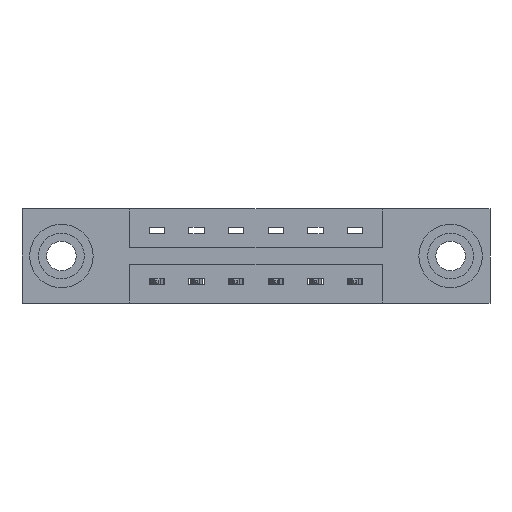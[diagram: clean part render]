
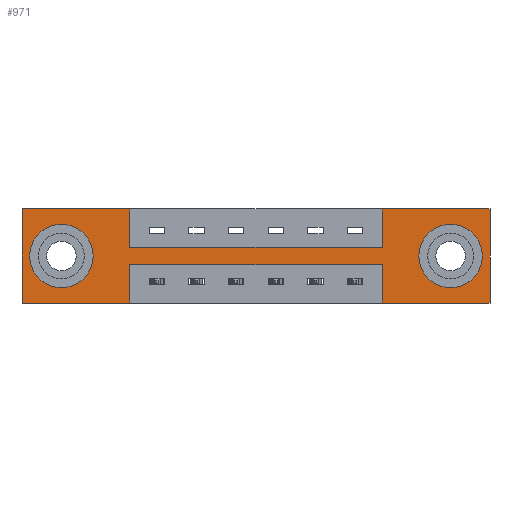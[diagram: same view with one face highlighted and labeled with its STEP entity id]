
A CAD part, front view. The second image highlights one B-rep face of the part: STEP entity #971.
In plain terms, the highlighted planar face has unit normal (0, -1, 0).
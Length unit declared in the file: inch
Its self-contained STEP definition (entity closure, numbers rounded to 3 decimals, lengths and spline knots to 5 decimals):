
#93 = VERTEX_POINT ( 'NONE', #6717 ) ;
#382 = ORIENTED_EDGE ( 'NONE', *, *, #2997, .F. ) ;
#542 = CARTESIAN_POINT ( 'NONE',  ( 1.417, 0., -0.15 ) ) ;
#563 = CARTESIAN_POINT ( 'NONE',  ( 0., 0., 0. ) ) ;
#632 = ORIENTED_EDGE ( 'NONE', *, *, #7686, .F. ) ;
#681 = EDGE_CURVE ( 'NONE', #6201, #2910, #5666, .T. ) ;
#719 = VERTEX_POINT ( 'NONE', #2175 ) ;
#766 = VERTEX_POINT ( 'NONE', #2208 ) ;
#838 = CIRCLE ( 'NONE', #7236, 0.078 ) ;
#924 = DIRECTION ( 'NONE',  ( 0., 0., -1. ) ) ;
#966 = CARTESIAN_POINT ( 'NONE',  ( 0., 0., -0.37 ) ) ;
#971 = ADVANCED_FACE ( 'NONE', ( #6395, #4572, #4335 ), #6551, .T. ) ;
#978 = LINE ( 'NONE', #7588, #6857 ) ;
#1150 = ORIENTED_EDGE ( 'NONE', *, *, #3278, .F. ) ;
#1361 = CARTESIAN_POINT ( 'NONE',  ( 0., 0., -0.37 ) ) ;
#1378 = VECTOR ( 'NONE', #2940, 39.37008 ) ;
#1530 = VECTOR ( 'NONE', #6991, 39.37008 ) ;
#1638 = VERTEX_POINT ( 'NONE', #3709 ) ;
#1661 = LINE ( 'NONE', #4416, #9433 ) ;
#1766 = VERTEX_POINT ( 'NONE', #563 ) ;
#1790 = ORIENTED_EDGE ( 'NONE', *, *, #7846, .T. ) ;
#2175 = CARTESIAN_POINT ( 'NONE',  ( 1.687, 0., -0.263 ) ) ;
#2208 = CARTESIAN_POINT ( 'NONE',  ( 0.425, 0., 0. ) ) ;
#2293 = VERTEX_POINT ( 'NONE', #4130 ) ;
#2416 = EDGE_CURVE ( 'NONE', #2293, #6888, #8305, .T. ) ;
#2449 = CARTESIAN_POINT ( 'NONE',  ( 1.687, 0., -0.185 ) ) ;
#2463 = CARTESIAN_POINT ( 'NONE',  ( 0.425, 0., 0. ) ) ;
#2646 = AXIS2_PLACEMENT_3D ( 'NONE', #8752, #4324, #9382 ) ;
#2883 = VERTEX_POINT ( 'NONE', #5233 ) ;
#2889 = CARTESIAN_POINT ( 'NONE',  ( 0.425, 0., -0.37 ) ) ;
#2910 = VERTEX_POINT ( 'NONE', #4475 ) ;
#2940 = DIRECTION ( 'NONE',  ( 0., 0., -1. ) ) ;
#2997 = EDGE_CURVE ( 'NONE', #1638, #3230, #7172, .T. ) ;
#3005 = LINE ( 'NONE', #4258, #5102 ) ;
#3043 = DIRECTION ( 'NONE',  ( 0., 1., 0. ) ) ;
#3058 = VECTOR ( 'NONE', #3884, 39.37008 ) ;
#3084 = LINE ( 'NONE', #4620, #8620 ) ;
#3142 = ORIENTED_EDGE ( 'NONE', *, *, #7053, .F. ) ;
#3230 = VERTEX_POINT ( 'NONE', #4614 ) ;
#3278 = EDGE_CURVE ( 'NONE', #2910, #93, #7640, .T. ) ;
#3315 = DIRECTION ( 'NONE',  ( 0., 0., -1. ) ) ;
#3488 = VERTEX_POINT ( 'NONE', #7374 ) ;
#3643 = CARTESIAN_POINT ( 'NONE',  ( 0.425, 0., -0.15 ) ) ;
#3709 = CARTESIAN_POINT ( 'NONE',  ( 1.842, 0., -0.37 ) ) ;
#3752 = LINE ( 'NONE', #9017, #9332 ) ;
#3884 = DIRECTION ( 'NONE',  ( -1., 0., 0. ) ) ;
#4019 = ORIENTED_EDGE ( 'NONE', *, *, #9321, .T. ) ;
#4111 = CIRCLE ( 'NONE', #8844, 0.078 ) ;
#4130 = CARTESIAN_POINT ( 'NONE',  ( 0.425, 0., -0.15 ) ) ;
#4258 = CARTESIAN_POINT ( 'NONE',  ( 1.842, 0., 0. ) ) ;
#4324 = DIRECTION ( 'NONE',  ( 0., 1., 0. ) ) ;
#4335 = FACE_OUTER_BOUND ( 'NONE', #8617, .T. ) ;
#4416 = CARTESIAN_POINT ( 'NONE',  ( 0., 0., 0. ) ) ;
#4475 = CARTESIAN_POINT ( 'NONE',  ( 0.425, 0., -0.37 ) ) ;
#4486 = ORIENTED_EDGE ( 'NONE', *, *, #8259, .F. ) ;
#4570 = CARTESIAN_POINT ( 'NONE',  ( 0.155, 0., -0.107 ) ) ;
#4572 = FACE_BOUND ( 'NONE', #6260, .T. ) ;
#4614 = CARTESIAN_POINT ( 'NONE',  ( 1.417, 0., -0.37 ) ) ;
#4620 = CARTESIAN_POINT ( 'NONE',  ( 0., 0., 0. ) ) ;
#4646 = CARTESIAN_POINT ( 'NONE',  ( 0.155, 0., -0.185 ) ) ;
#4681 = EDGE_CURVE ( 'NONE', #8097, #1638, #3005, .T. ) ;
#4729 = ORIENTED_EDGE ( 'NONE', *, *, #4681, .F. ) ;
#4920 = AXIS2_PLACEMENT_3D ( 'NONE', #4646, #9637, #5434 ) ;
#5102 = VECTOR ( 'NONE', #924, 39.37008 ) ;
#5192 = DIRECTION ( 'NONE',  ( 0., 0., 1. ) ) ;
#5233 = CARTESIAN_POINT ( 'NONE',  ( 1.417, 0., -0.22 ) ) ;
#5306 = EDGE_CURVE ( 'NONE', #93, #1766, #1661, .T. ) ;
#5434 = DIRECTION ( 'NONE',  ( 0., 0., 1. ) ) ;
#5518 = EDGE_CURVE ( 'NONE', #7432, #8097, #7824, .T. ) ;
#5534 = AXIS2_PLACEMENT_3D ( 'NONE', #966, #6732, #7203 ) ;
#5666 = LINE ( 'NONE', #2889, #1378 ) ;
#5799 = VECTOR ( 'NONE', #9416, 39.37008 ) ;
#5959 = VERTEX_POINT ( 'NONE', #6008 ) ;
#6008 = CARTESIAN_POINT ( 'NONE',  ( 0.155, 0., -0.263 ) ) ;
#6182 = DIRECTION ( 'NONE',  ( 1., 0., 0. ) ) ;
#6201 = VERTEX_POINT ( 'NONE', #7840 ) ;
#6251 = CARTESIAN_POINT ( 'NONE',  ( 0., 0., 0. ) ) ;
#6260 = EDGE_LOOP ( 'NONE', ( #4019, #8054 ) ) ;
#6314 = ORIENTED_EDGE ( 'NONE', *, *, #681, .F. ) ;
#6357 = VECTOR ( 'NONE', #8537, 39.37008 ) ;
#6392 = CARTESIAN_POINT ( 'NONE',  ( 0., 0., -0.37 ) ) ;
#6395 = FACE_BOUND ( 'NONE', #6720, .T. ) ;
#6533 = LINE ( 'NONE', #2463, #8046 ) ;
#6551 = PLANE ( 'NONE',  #5534 ) ;
#6717 = CARTESIAN_POINT ( 'NONE',  ( 0., 0., -0.37 ) ) ;
#6720 = EDGE_LOOP ( 'NONE', ( #9536, #1790 ) ) ;
#6732 = DIRECTION ( 'NONE',  ( 0., -1., 0. ) ) ;
#6829 = DIRECTION ( 'NONE',  ( -1., 0., 0. ) ) ;
#6857 = VECTOR ( 'NONE', #8293, 39.37008 ) ;
#6888 = VERTEX_POINT ( 'NONE', #542 ) ;
#6991 = DIRECTION ( 'NONE',  ( 1., 0., 0. ) ) ;
#7053 = EDGE_CURVE ( 'NONE', #766, #2293, #6533, .T. ) ;
#7171 = DIRECTION ( 'NONE',  ( 0., 0., -1. ) ) ;
#7172 = LINE ( 'NONE', #6392, #3058 ) ;
#7203 = DIRECTION ( 'NONE',  ( 0., 0., -1. ) ) ;
#7236 = AXIS2_PLACEMENT_3D ( 'NONE', #7669, #3043, #8364 ) ;
#7254 = ORIENTED_EDGE ( 'NONE', *, *, #9725, .F. ) ;
#7374 = CARTESIAN_POINT ( 'NONE',  ( 1.687, 0., -0.107 ) ) ;
#7403 = CARTESIAN_POINT ( 'NONE',  ( 1.417, 0., -0.37 ) ) ;
#7414 = VECTOR ( 'NONE', #6829, 39.37008 ) ;
#7432 = VERTEX_POINT ( 'NONE', #9423 ) ;
#7588 = CARTESIAN_POINT ( 'NONE',  ( 0.425, 0., -0.22 ) ) ;
#7640 = LINE ( 'NONE', #1361, #7414 ) ;
#7669 = CARTESIAN_POINT ( 'NONE',  ( 1.687, 0., -0.185 ) ) ;
#7685 = EDGE_CURVE ( 'NONE', #5959, #8290, #9523, .T. ) ;
#7686 = EDGE_CURVE ( 'NONE', #6888, #7432, #3752, .T. ) ;
#7824 = LINE ( 'NONE', #6251, #1530 ) ;
#7840 = CARTESIAN_POINT ( 'NONE',  ( 0.425, 0., -0.22 ) ) ;
#7846 = EDGE_CURVE ( 'NONE', #719, #3488, #4111, .T. ) ;
#7912 = DIRECTION ( 'NONE',  ( 0., 1., 0. ) ) ;
#8046 = VECTOR ( 'NONE', #7171, 39.37008 ) ;
#8054 = ORIENTED_EDGE ( 'NONE', *, *, #7685, .T. ) ;
#8097 = VERTEX_POINT ( 'NONE', #9394 ) ;
#8156 = EDGE_CURVE ( 'NONE', #3230, #2883, #9516, .T. ) ;
#8259 = EDGE_CURVE ( 'NONE', #2883, #6201, #978, .T. ) ;
#8290 = VERTEX_POINT ( 'NONE', #4570 ) ;
#8293 = DIRECTION ( 'NONE',  ( -1., 0., 0. ) ) ;
#8305 = LINE ( 'NONE', #3643, #6357 ) ;
#8364 = DIRECTION ( 'NONE',  ( 0., 0., -1. ) ) ;
#8386 = DIRECTION ( 'NONE',  ( 0., 0., 1. ) ) ;
#8464 = ORIENTED_EDGE ( 'NONE', *, *, #8156, .F. ) ;
#8537 = DIRECTION ( 'NONE',  ( 1., 0., 0. ) ) ;
#8617 = EDGE_LOOP ( 'NONE', ( #6314, #4486, #8464, #382, #4729, #8665, #632, #8861, #3142, #7254, #9055, #1150 ) ) ;
#8620 = VECTOR ( 'NONE', #6182, 39.37008 ) ;
#8665 = ORIENTED_EDGE ( 'NONE', *, *, #5518, .F. ) ;
#8729 = CIRCLE ( 'NONE', #2646, 0.078 ) ;
#8752 = CARTESIAN_POINT ( 'NONE',  ( 0.155, 0., -0.185 ) ) ;
#8844 = AXIS2_PLACEMENT_3D ( 'NONE', #2449, #7912, #3315 ) ;
#8861 = ORIENTED_EDGE ( 'NONE', *, *, #2416, .F. ) ;
#9017 = CARTESIAN_POINT ( 'NONE',  ( 1.417, 0., 0. ) ) ;
#9055 = ORIENTED_EDGE ( 'NONE', *, *, #5306, .F. ) ;
#9105 = EDGE_CURVE ( 'NONE', #3488, #719, #838, .T. ) ;
#9321 = EDGE_CURVE ( 'NONE', #8290, #5959, #8729, .T. ) ;
#9332 = VECTOR ( 'NONE', #8386, 39.37008 ) ;
#9382 = DIRECTION ( 'NONE',  ( 0., 0., 1. ) ) ;
#9394 = CARTESIAN_POINT ( 'NONE',  ( 1.842, 0., 0. ) ) ;
#9416 = DIRECTION ( 'NONE',  ( 0., 0., 1. ) ) ;
#9423 = CARTESIAN_POINT ( 'NONE',  ( 1.417, 0., 0. ) ) ;
#9433 = VECTOR ( 'NONE', #5192, 39.37008 ) ;
#9516 = LINE ( 'NONE', #7403, #5799 ) ;
#9523 = CIRCLE ( 'NONE', #4920, 0.078 ) ;
#9536 = ORIENTED_EDGE ( 'NONE', *, *, #9105, .T. ) ;
#9637 = DIRECTION ( 'NONE',  ( 0., 1., 0. ) ) ;
#9725 = EDGE_CURVE ( 'NONE', #1766, #766, #3084, .T. ) ;
